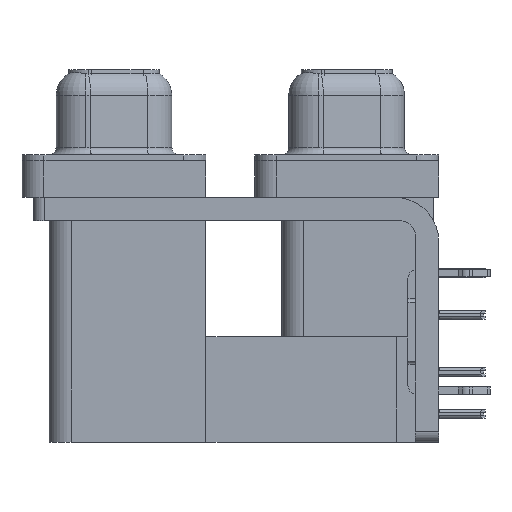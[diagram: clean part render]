
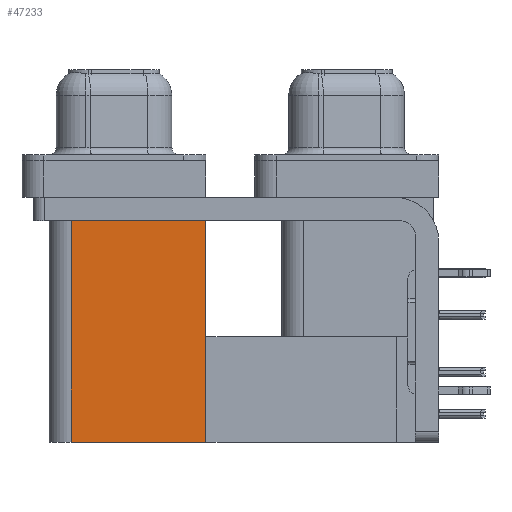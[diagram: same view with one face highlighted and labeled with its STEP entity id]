
A CAD part, left-side view. The second image highlights one B-rep face of the part: STEP entity #47233.
In plain terms, the highlighted planar face has unit normal (-1, 0, 0).
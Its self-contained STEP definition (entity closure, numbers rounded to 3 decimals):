
#767 = EDGE_LOOP ( 'NONE', ( #2888, #26583, #20164, #45359 ) ) ;
#2888 = ORIENTED_EDGE ( 'NONE', *, *, #38053, .T. ) ;
#7608 = CARTESIAN_POINT ( 'NONE',  ( 3.765, 9.6, -2.5 ) ) ;
#9721 = CARTESIAN_POINT ( 'NONE',  ( 3.765, 9.6, -19.2 ) ) ;
#14289 = DIRECTION ( 'NONE',  ( 0., 0., 1. ) ) ;
#15059 = LINE ( 'NONE', #34050, #30510 ) ;
#20097 = LINE ( 'NONE', #44244, #36860 ) ;
#20164 = ORIENTED_EDGE ( 'NONE', *, *, #20254, .F. ) ;
#20254 = EDGE_CURVE ( 'NONE', #32007, #41595, #28320, .T. ) ;
#24751 = DIRECTION ( 'NONE',  ( 0., 0., 1. ) ) ;
#26139 = AXIS2_PLACEMENT_3D ( 'NONE', #9721, #45327, #41451 ) ;
#26583 = ORIENTED_EDGE ( 'NONE', *, *, #32567, .F. ) ;
#27873 = VECTOR ( 'NONE', #28569, 1000. ) ;
#28059 = CARTESIAN_POINT ( 'NONE',  ( 3.765, 9.6, -19.2 ) ) ;
#28320 = LINE ( 'NONE', #28059, #27873 ) ;
#28569 = DIRECTION ( 'NONE',  ( 0., 1., 0. ) ) ;
#30405 = VERTEX_POINT ( 'NONE', #7608 ) ;
#30510 = VECTOR ( 'NONE', #14289, 1000. ) ;
#32007 = VERTEX_POINT ( 'NONE', #40229 ) ;
#32567 = EDGE_CURVE ( 'NONE', #41595, #32739, #20097, .T. ) ;
#32739 = VERTEX_POINT ( 'NONE', #50754 ) ;
#33394 = FACE_OUTER_BOUND ( 'NONE', #767, .T. ) ;
#34050 = CARTESIAN_POINT ( 'NONE',  ( 3.765, 9.6, -19.2 ) ) ;
#36428 = EDGE_CURVE ( 'NONE', #32007, #30405, #15059, .T. ) ;
#36776 = CARTESIAN_POINT ( 'NONE',  ( 3.765, 18.8, -19.2 ) ) ;
#36860 = VECTOR ( 'NONE', #24751, 1000. ) ;
#38053 = EDGE_CURVE ( 'NONE', #30405, #32739, #42805, .T. ) ;
#40229 = CARTESIAN_POINT ( 'NONE',  ( 3.765, 9.6, -19.2 ) ) ;
#41413 = VECTOR ( 'NONE', #42040, 1000. ) ;
#41451 = DIRECTION ( 'NONE',  ( 0., 0., -1. ) ) ;
#41595 = VERTEX_POINT ( 'NONE', #36776 ) ;
#42040 = DIRECTION ( 'NONE',  ( 0., 1., 0. ) ) ;
#42805 = LINE ( 'NONE', #46446, #41413 ) ;
#44244 = CARTESIAN_POINT ( 'NONE',  ( 3.765, 18.8, -19.2 ) ) ;
#45327 = DIRECTION ( 'NONE',  ( 1., 0., 0. ) ) ;
#45359 = ORIENTED_EDGE ( 'NONE', *, *, #36428, .T. ) ;
#46446 = CARTESIAN_POINT ( 'NONE',  ( 3.765, 9.6, -2.5 ) ) ;
#47233 = ADVANCED_FACE ( 'NONE', ( #33394 ), #49766, .F. ) ;
#49766 = PLANE ( 'NONE',  #26139 ) ;
#50754 = CARTESIAN_POINT ( 'NONE',  ( 3.765, 18.8, -2.5 ) ) ;
